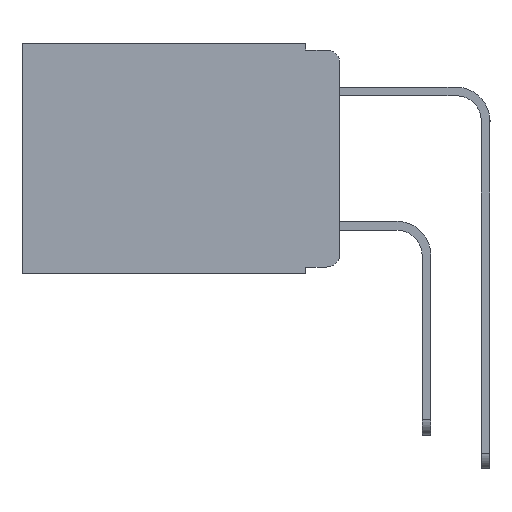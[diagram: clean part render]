
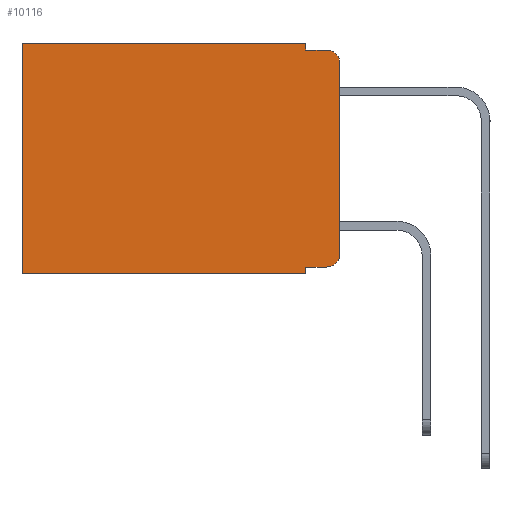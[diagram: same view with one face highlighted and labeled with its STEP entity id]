
A CAD part, left-side view. The second image highlights one B-rep face of the part: STEP entity #10116.
In plain terms, the highlighted planar face has unit normal (-1, 0, 0).
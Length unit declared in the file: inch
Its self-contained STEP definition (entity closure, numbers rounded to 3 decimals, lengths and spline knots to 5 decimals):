
#167 = VECTOR ( 'NONE', #5252, 39.37008 ) ;
#436 = CARTESIAN_POINT ( 'NONE',  ( 0.298, 0.051, 0. ) ) ;
#506 = LINE ( 'NONE', #10190, #167 ) ;
#569 = VECTOR ( 'NONE', #11071, 39.37008 ) ;
#877 = CARTESIAN_POINT ( 'NONE',  ( 0.298, 0.02, -0.01 ) ) ;
#963 = AXIS2_PLACEMENT_3D ( 'NONE', #3617, #6121, #7937 ) ;
#1110 = VECTOR ( 'NONE', #2199, 39.37008 ) ;
#1193 = VERTEX_POINT ( 'NONE', #8121 ) ;
#1436 = DIRECTION ( 'NONE',  ( 1., 0., 0. ) ) ;
#1526 = DIRECTION ( 'NONE',  ( 0., 0., -1. ) ) ;
#1567 = EDGE_CURVE ( 'NONE', #6526, #5903, #11236, .T. ) ;
#1698 = AXIS2_PLACEMENT_3D ( 'NONE', #12563, #1436, #8767 ) ;
#1706 = DIRECTION ( 'NONE',  ( 0., 0., -1. ) ) ;
#2089 = ORIENTED_EDGE ( 'NONE', *, *, #11728, .T. ) ;
#2199 = DIRECTION ( 'NONE',  ( 0., 1., 0. ) ) ;
#2486 = EDGE_CURVE ( 'NONE', #9372, #5362, #5589, .T. ) ;
#2770 = CARTESIAN_POINT ( 'NONE',  ( 0.298, 0.473, 0. ) ) ;
#2815 = ORIENTED_EDGE ( 'NONE', *, *, #12984, .T. ) ;
#2937 = CARTESIAN_POINT ( 'NONE',  ( 0.298, 0.051, -0.343 ) ) ;
#3401 = CARTESIAN_POINT ( 'NONE',  ( 0.298, 0.051, -0.01 ) ) ;
#3523 = LINE ( 'NONE', #4079, #569 ) ;
#3583 = CARTESIAN_POINT ( 'NONE',  ( 0.298, 0.473, 0. ) ) ;
#3617 = CARTESIAN_POINT ( 'NONE',  ( 0.298, 0.02, -0.03 ) ) ;
#3688 = DIRECTION ( 'NONE',  ( 0., 0., -1. ) ) ;
#3721 = EDGE_CURVE ( 'NONE', #5903, #1193, #9889, .T. ) ;
#4069 = FACE_OUTER_BOUND ( 'NONE', #6818, .T. ) ;
#4079 = CARTESIAN_POINT ( 'NONE',  ( 0.298, 0.051, -0.333 ) ) ;
#4491 = ORIENTED_EDGE ( 'NONE', *, *, #4697, .F. ) ;
#4697 = EDGE_CURVE ( 'NONE', #12666, #5362, #4862, .T. ) ;
#4718 = PLANE ( 'NONE',  #1698 ) ;
#4843 = ORIENTED_EDGE ( 'NONE', *, *, #1567, .T. ) ;
#4862 = LINE ( 'NONE', #3401, #12372 ) ;
#5106 = DIRECTION ( 'NONE',  ( -1., 0., 0. ) ) ;
#5189 = ORIENTED_EDGE ( 'NONE', *, *, #3721, .T. ) ;
#5211 = VERTEX_POINT ( 'NONE', #12553 ) ;
#5252 = DIRECTION ( 'NONE',  ( 0., 0., -1. ) ) ;
#5362 = VERTEX_POINT ( 'NONE', #877 ) ;
#5518 = ORIENTED_EDGE ( 'NONE', *, *, #10576, .F. ) ;
#5589 = CIRCLE ( 'NONE', #963, 0.02 ) ;
#5903 = VERTEX_POINT ( 'NONE', #2770 ) ;
#6054 = VECTOR ( 'NONE', #12542, 39.37008 ) ;
#6121 = DIRECTION ( 'NONE',  ( -1., 0., 0. ) ) ;
#6526 = VERTEX_POINT ( 'NONE', #6947 ) ;
#6565 = LINE ( 'NONE', #436, #8884 ) ;
#6818 = EDGE_LOOP ( 'NONE', ( #8930, #6920, #4491, #7235, #4843, #5189, #5518, #9695, #2089, #2815 ) ) ;
#6911 = CIRCLE ( 'NONE', #10440, 0.02 ) ;
#6920 = ORIENTED_EDGE ( 'NONE', *, *, #2486, .T. ) ;
#6947 = CARTESIAN_POINT ( 'NONE',  ( 0.298, 0.051, 0. ) ) ;
#7235 = ORIENTED_EDGE ( 'NONE', *, *, #7447, .F. ) ;
#7374 = CARTESIAN_POINT ( 'NONE',  ( 0.298, 0., 0. ) ) ;
#7447 = EDGE_CURVE ( 'NONE', #6526, #12666, #506, .T. ) ;
#7543 = CARTESIAN_POINT ( 'NONE',  ( 0.298, 0.051, -0.01 ) ) ;
#7797 = CARTESIAN_POINT ( 'NONE',  ( 0.298, 0., 0. ) ) ;
#7864 = EDGE_CURVE ( 'NONE', #5211, #12378, #6565, .T. ) ;
#7937 = DIRECTION ( 'NONE',  ( 0., 0., -1. ) ) ;
#8121 = CARTESIAN_POINT ( 'NONE',  ( 0.298, 0.473, -0.343 ) ) ;
#8462 = CARTESIAN_POINT ( 'NONE',  ( 0.298, 0., -0.343 ) ) ;
#8766 = LINE ( 'NONE', #7797, #11319 ) ;
#8767 = DIRECTION ( 'NONE',  ( 0., 0., -1. ) ) ;
#8884 = VECTOR ( 'NONE', #1526, 39.37008 ) ;
#8930 = ORIENTED_EDGE ( 'NONE', *, *, #12825, .F. ) ;
#9140 = LINE ( 'NONE', #8462, #1110 ) ;
#9308 = VERTEX_POINT ( 'NONE', #13106 ) ;
#9372 = VERTEX_POINT ( 'NONE', #9425 ) ;
#9425 = CARTESIAN_POINT ( 'NONE',  ( 0.298, 0., -0.03 ) ) ;
#9695 = ORIENTED_EDGE ( 'NONE', *, *, #7864, .F. ) ;
#9889 = LINE ( 'NONE', #3583, #12396 ) ;
#10116 = ADVANCED_FACE ( 'NONE', ( #4069 ), #4718, .F. ) ;
#10190 = CARTESIAN_POINT ( 'NONE',  ( 0.298, 0.051, 0. ) ) ;
#10440 = AXIS2_PLACEMENT_3D ( 'NONE', #11004, #5106, #11946 ) ;
#10576 = EDGE_CURVE ( 'NONE', #12378, #1193, #9140, .T. ) ;
#10837 = VERTEX_POINT ( 'NONE', #12639 ) ;
#11004 = CARTESIAN_POINT ( 'NONE',  ( 0.298, 0.02, -0.313 ) ) ;
#11071 = DIRECTION ( 'NONE',  ( 0., -1., 0. ) ) ;
#11236 = LINE ( 'NONE', #7374, #6054 ) ;
#11319 = VECTOR ( 'NONE', #3688, 39.37008 ) ;
#11728 = EDGE_CURVE ( 'NONE', #5211, #10837, #3523, .T. ) ;
#11946 = DIRECTION ( 'NONE',  ( 0., 0., -1. ) ) ;
#12058 = DIRECTION ( 'NONE',  ( 0., -1., 0. ) ) ;
#12372 = VECTOR ( 'NONE', #12058, 39.37008 ) ;
#12378 = VERTEX_POINT ( 'NONE', #2937 ) ;
#12396 = VECTOR ( 'NONE', #1706, 39.37008 ) ;
#12542 = DIRECTION ( 'NONE',  ( 0., 1., 0. ) ) ;
#12553 = CARTESIAN_POINT ( 'NONE',  ( 0.298, 0.051, -0.333 ) ) ;
#12563 = CARTESIAN_POINT ( 'NONE',  ( 0.298, 0., 0. ) ) ;
#12639 = CARTESIAN_POINT ( 'NONE',  ( 0.298, 0.02, -0.333 ) ) ;
#12666 = VERTEX_POINT ( 'NONE', #7543 ) ;
#12825 = EDGE_CURVE ( 'NONE', #9372, #9308, #8766, .T. ) ;
#12984 = EDGE_CURVE ( 'NONE', #10837, #9308, #6911, .T. ) ;
#13106 = CARTESIAN_POINT ( 'NONE',  ( 0.298, 0., -0.313 ) ) ;
